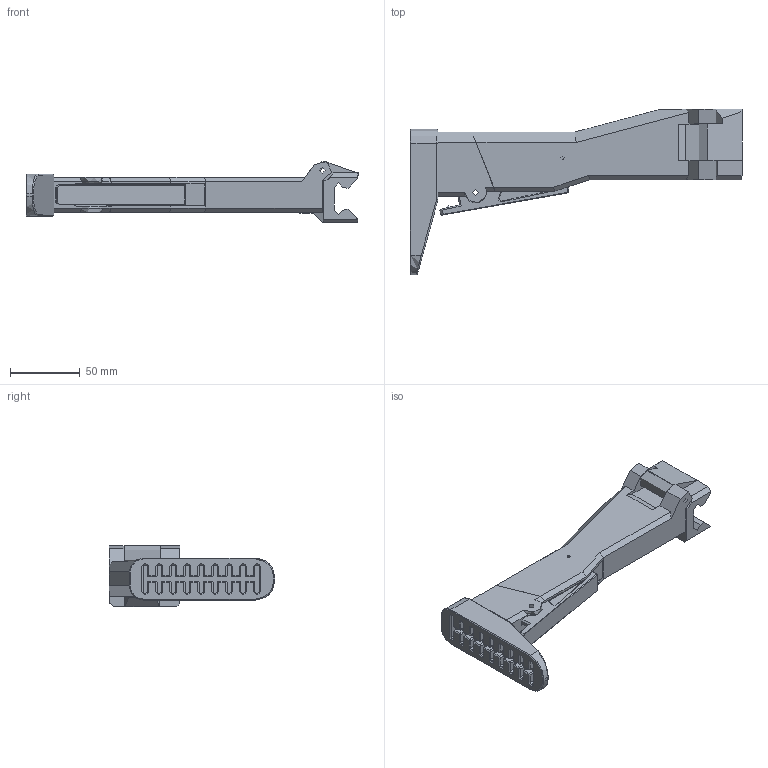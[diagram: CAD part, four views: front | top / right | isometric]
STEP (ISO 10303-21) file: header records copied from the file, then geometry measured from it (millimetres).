
FILE_DESCRIPTION(/* description */ (''),/* implementation_level */ '2;1');
FILE_NAME(/* name */ 'evo3.stp',/* time_stamp */ '2021-01-23T20:20:46+02:00',/* author */ (''),/* organization */ (''),/* preprocessor_version */ 'ST-DEVELOPER v15.2',/* originating_system */ 'Autodesk Translator Framework v2.0.0.5431',/* authorisation */ '');
FILE_SCHEMA (('AUTOMOTIVE_DESIGN { 1 0 10303 214 3 1 1 }'));
Length unit declared in the file: centimetre
Products named in the file (1): (Unsaved)
Bounding box: 237.32 x 118.38 x 43.89 mm (x, y, z)
Volume: 265657.2 mm3; surface area: 93857 mm2
Topology: 7 solids, 7 shells, 763 faces, 1975 edges, 1245 vertices
Faces by surface type: plane 480, cylinder 161, cone 82, bspline 22, torus 16, sphere 2
Full cylindrical faces by diameter (mm): 2.2 x2, 2.6 x1, 3 x2, 4 x3, 4.4 x4, 6.4 x1, 6.6 x1, 7 x1, 12.1 x1, 20.5 x1
Entity records: 23644 total; most frequent: CARTESIAN_POINT 4885, ORIENTED_EDGE 3900, DIRECTION 3844, EDGE_CURVE 1950, LINE 1436, VECTOR 1436, VERTEX_POINT 1240, AXIS2_PLACEMENT_3D 1204
